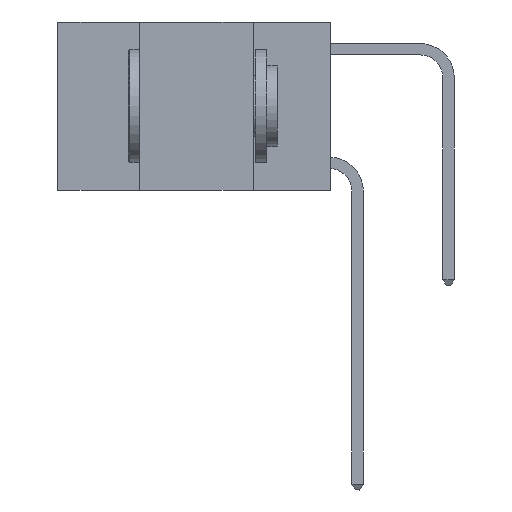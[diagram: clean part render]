
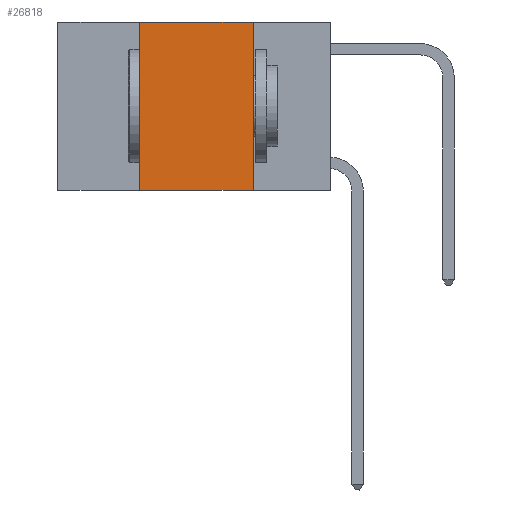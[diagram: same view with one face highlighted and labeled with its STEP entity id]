
A CAD part, left-side view. The second image highlights one B-rep face of the part: STEP entity #26818.
In plain terms, the highlighted planar face has unit normal (-1, 0, 0).
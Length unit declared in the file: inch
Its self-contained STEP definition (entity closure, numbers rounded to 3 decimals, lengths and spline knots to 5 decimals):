
#100 = LINE ( 'NONE', #9881, #2607 ) ;
#872 = DIRECTION ( 'NONE',  ( 0., -1., 0. ) ) ;
#2607 = VECTOR ( 'NONE', #872, 39.37008 ) ;
#3568 = CARTESIAN_POINT ( 'NONE',  ( 0., 0.17, 0. ) ) ;
#5195 = EDGE_CURVE ( 'NONE', #6880, #14353, #26376, .T. ) ;
#6880 = VERTEX_POINT ( 'NONE', #6944 ) ;
#6944 = CARTESIAN_POINT ( 'NONE',  ( 0., 0.17, 0. ) ) ;
#7540 = CARTESIAN_POINT ( 'NONE',  ( 0., 0.6, -0.37 ) ) ;
#7992 = CARTESIAN_POINT ( 'NONE',  ( 0., 0.6, 0. ) ) ;
#8842 = EDGE_CURVE ( 'NONE', #13119, #6880, #100, .T. ) ;
#9158 = EDGE_LOOP ( 'NONE', ( #10431, #14051, #23431, #23354 ) ) ;
#9721 = PLANE ( 'NONE',  #22895 ) ;
#9881 = CARTESIAN_POINT ( 'NONE',  ( 0., 0.6, 0. ) ) ;
#9884 = EDGE_CURVE ( 'NONE', #25704, #14353, #14855, .T. ) ;
#10266 = FACE_OUTER_BOUND ( 'NONE', #9158, .T. ) ;
#10431 = ORIENTED_EDGE ( 'NONE', *, *, #5195, .F. ) ;
#13043 = VECTOR ( 'NONE', #14432, 39.37008 ) ;
#13119 = VERTEX_POINT ( 'NONE', #13307 ) ;
#13307 = CARTESIAN_POINT ( 'NONE',  ( 0., 0.42, 0. ) ) ;
#14051 = ORIENTED_EDGE ( 'NONE', *, *, #8842, .F. ) ;
#14353 = VERTEX_POINT ( 'NONE', #19379 ) ;
#14432 = DIRECTION ( 'NONE',  ( 0., -1., 0. ) ) ;
#14855 = LINE ( 'NONE', #7540, #13043 ) ;
#15789 = CARTESIAN_POINT ( 'NONE',  ( 0., 0.42, 0. ) ) ;
#17845 = VECTOR ( 'NONE', #26581, 39.37008 ) ;
#19379 = CARTESIAN_POINT ( 'NONE',  ( 0., 0.17, -0.37 ) ) ;
#22533 = DIRECTION ( 'NONE',  ( 0., 0., 1. ) ) ;
#22895 = AXIS2_PLACEMENT_3D ( 'NONE', #7992, #28029, #23612 ) ;
#23354 = ORIENTED_EDGE ( 'NONE', *, *, #9884, .T. ) ;
#23431 = ORIENTED_EDGE ( 'NONE', *, *, #28923, .F. ) ;
#23612 = DIRECTION ( 'NONE',  ( 0., 0., -1. ) ) ;
#23965 = LINE ( 'NONE', #15789, #26479 ) ;
#25704 = VERTEX_POINT ( 'NONE', #28385 ) ;
#26376 = LINE ( 'NONE', #3568, #17845 ) ;
#26479 = VECTOR ( 'NONE', #22533, 39.37008 ) ;
#26581 = DIRECTION ( 'NONE',  ( 0., 0., -1. ) ) ;
#26818 = ADVANCED_FACE ( 'NONE', ( #10266 ), #9721, .F. ) ;
#28029 = DIRECTION ( 'NONE',  ( 1., 0., 0. ) ) ;
#28385 = CARTESIAN_POINT ( 'NONE',  ( 0., 0.42, -0.37 ) ) ;
#28923 = EDGE_CURVE ( 'NONE', #25704, #13119, #23965, .T. ) ;
